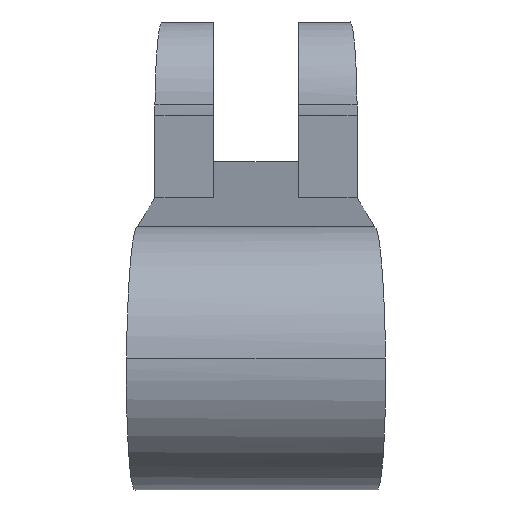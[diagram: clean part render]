
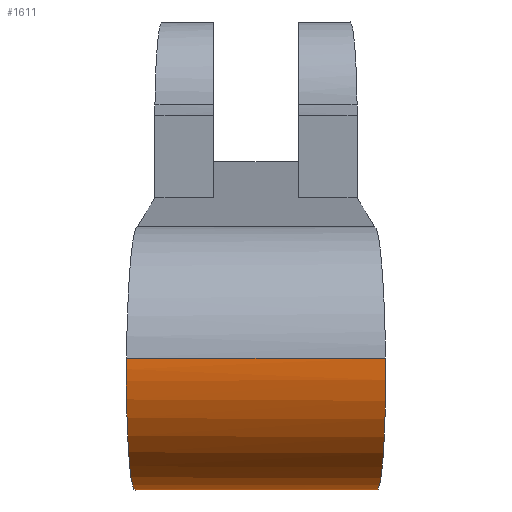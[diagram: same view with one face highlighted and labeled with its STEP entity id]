
A CAD part, top view. The second image highlights one B-rep face of the part: STEP entity #1611.
In plain terms, the highlighted cylindrical face has radius 5.625 mm (diameter 11.25 mm), a partial arc.
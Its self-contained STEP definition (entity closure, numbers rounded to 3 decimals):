
#6 = CARTESIAN_POINT ( 'NONE',  ( 12.383, -4.545, -4.303 ) ) ;
#8 = CARTESIAN_POINT ( 'NONE',  ( 12.698, -6.107, -0.244 ) ) ;
#21 = CARTESIAN_POINT ( 'NONE',  ( 12.94, -3.644, 3.341 ) ) ;
#23 = CARTESIAN_POINT ( 'NONE',  ( 2.363, -4.545, -4.303 ) ) ;
#27 = CARTESIAN_POINT ( 'NONE',  ( 2.363, -4.545, -4.303 ) ) ;
#29 = CARTESIAN_POINT ( 'NONE',  ( 12.9, 0.705, 3.341 ) ) ;
#53 = CARTESIAN_POINT ( 'NONE',  ( 1.847, 0.705, 3.341 ) ) ;
#73 = CARTESIAN_POINT ( 'NONE',  ( 2.048, -6.107, -0.244 ) ) ;
#161 = DIRECTION ( 'NONE',  ( -1., 0., 0. ) ) ;
#184 =( BOUNDED_CURVE ( )  B_SPLINE_CURVE ( 3, ( #27, #73, #617, #53 ),
 .UNSPECIFIED., .F., .F. ) 
 B_SPLINE_CURVE_WITH_KNOTS ( ( 4, 4 ),
 ( 4.47, 6.408 ),
 .UNSPECIFIED. ) 
 CURVE ( )  GEOMETRIC_REPRESENTATION_ITEM ( )  RATIONAL_B_SPLINE_CURVE ( ( 1., 0.711, 0.711, 1. ) ) 
 REPRESENTATION_ITEM ( '' )  );
#407 = VERTEX_POINT ( 'NONE', #703 ) ;
#455 = CARTESIAN_POINT ( 'NONE',  ( 12.9, 0.705, 3.341 ) ) ;
#460 = CARTESIAN_POINT ( 'NONE',  ( 12.903, -4.545, -4.303 ) ) ;
#473 = VECTOR ( 'NONE', #161, 1000. ) ;
#477 = VERTEX_POINT ( 'NONE', #455 ) ;
#495 = LINE ( 'NONE', #460, #473 ) ;
#537 = VECTOR ( 'NONE', #1149, 1000. ) ;
#564 = LINE ( 'NONE', #1390, #537 ) ;
#566 = DIRECTION ( 'NONE',  ( -1., 0., 0. ) ) ;
#586 = ORIENTED_EDGE ( 'NONE', *, *, #765, .F. ) ;
#594 = ORIENTED_EDGE ( 'NONE', *, *, #800, .T. ) ;
#617 = CARTESIAN_POINT ( 'NONE',  ( 1.806, -3.644, 3.341 ) ) ;
#625 = ORIENTED_EDGE ( 'NONE', *, *, #801, .F. ) ;
#703 = CARTESIAN_POINT ( 'NONE',  ( 1.847, 0.705, 3.341 ) ) ;
#765 = EDGE_CURVE ( 'NONE', #477, #1382, #1625, .T. ) ;
#782 = ORIENTED_EDGE ( 'NONE', *, *, #828, .F. ) ;
#800 = EDGE_CURVE ( 'NONE', #477, #407, #564, .T. ) ;
#801 = EDGE_CURVE ( 'NONE', #992, #407, #184, .T. ) ;
#828 = EDGE_CURVE ( 'NONE', #1382, #992, #495, .T. ) ;
#920 = CYLINDRICAL_SURFACE ( 'NONE', #923, 5.625 ) ;
#923 = AXIS2_PLACEMENT_3D ( 'NONE', #1464, #566, #1267 ) ;
#935 = FACE_OUTER_BOUND ( 'NONE', #1567, .T. ) ;
#992 = VERTEX_POINT ( 'NONE', #23 ) ;
#1149 = DIRECTION ( 'NONE',  ( -1., 0., 0. ) ) ;
#1267 = DIRECTION ( 'NONE',  ( 0., 0., 1. ) ) ;
#1367 = CARTESIAN_POINT ( 'NONE',  ( 12.383, -4.545, -4.303 ) ) ;
#1382 = VERTEX_POINT ( 'NONE', #1367 ) ;
#1390 = CARTESIAN_POINT ( 'NONE',  ( 12.903, 0.705, 3.341 ) ) ;
#1464 = CARTESIAN_POINT ( 'NONE',  ( 12.903, 0.705, -2.284 ) ) ;
#1567 = EDGE_LOOP ( 'NONE', ( #586, #594, #625, #782 ) ) ;
#1611 = ADVANCED_FACE ( 'NONE', ( #935 ), #920, .T. ) ;
#1625 =( BOUNDED_CURVE ( )  B_SPLINE_CURVE ( 3, ( #29, #21, #8, #6 ),
 .UNSPECIFIED., .F., .F. ) 
 B_SPLINE_CURVE_WITH_KNOTS ( ( 4, 4 ),
 ( 3.017, 4.955 ),
 .UNSPECIFIED. ) 
 CURVE ( )  GEOMETRIC_REPRESENTATION_ITEM ( )  RATIONAL_B_SPLINE_CURVE ( ( 1., 0.711, 0.711, 1. ) ) 
 REPRESENTATION_ITEM ( '' )  );
